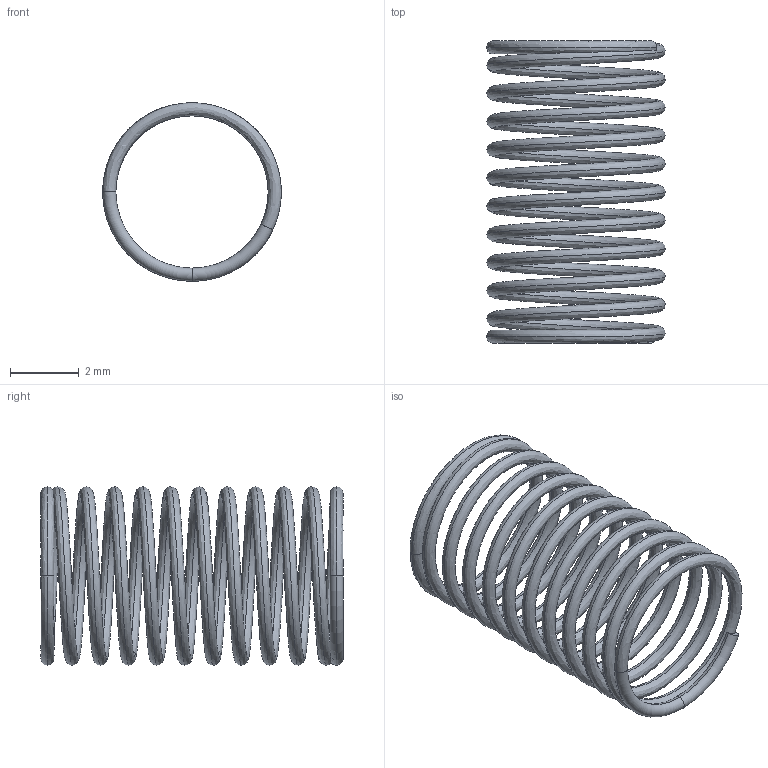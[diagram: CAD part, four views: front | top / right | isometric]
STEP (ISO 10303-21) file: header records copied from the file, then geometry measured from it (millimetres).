
FILE_DESCRIPTION (( 'STEP AP214' ), '1' );
FILE_NAME ('Firing Pin Spring.step', '2014-07-30T19:45:45', ( 'WarFairy' ), ( '' ), 'SwSTEP 2.0', 'SolidWorks 2013', '' );
FILE_SCHEMA (( 'AUTOMOTIVE_DESIGN' ));
Length unit declared in the file: millimetre
Products named in the file (1): Firing Pin Spring
Bounding box: 5.19 x 8.79 x 5.19 mm (x, y, z)
Volume: 20.3 mm3; surface area: 210.3 mm2
Topology: 1 solids, 1 shells, 11 faces, 27 edges, 16 vertices
Faces by surface type: torus 5, bspline 4, plane 2
Entity records: 4943 total; most frequent: CARTESIAN_POINT 4683, ORIENTED_EDGE 54, DIRECTION 36, EDGE_CURVE 27, AXIS2_PLACEMENT_3D 18, VERTEX_POINT 16, B_SPLINE_CURVE_WITH_KNOTS 15, EDGE_LOOP 13
